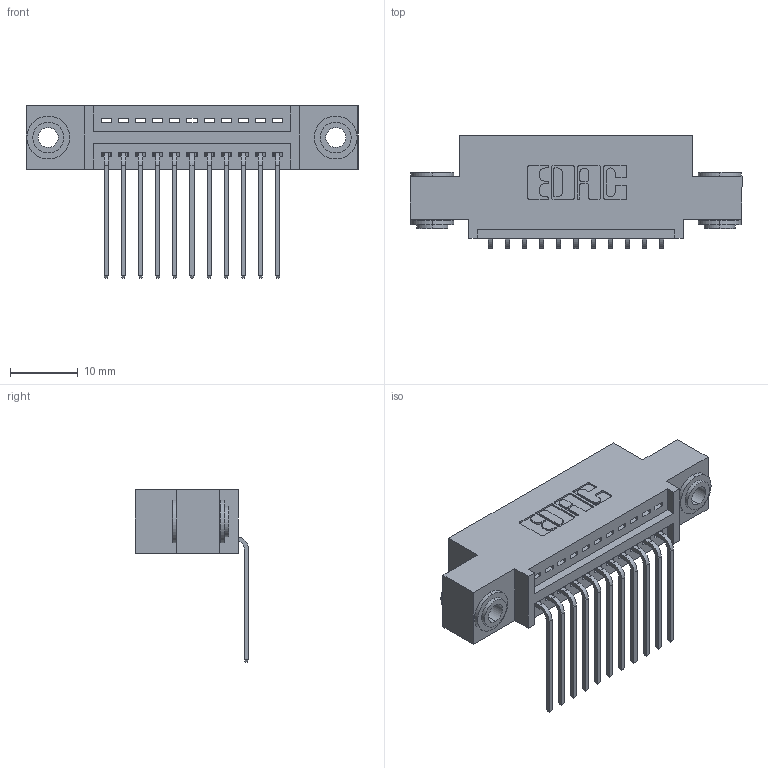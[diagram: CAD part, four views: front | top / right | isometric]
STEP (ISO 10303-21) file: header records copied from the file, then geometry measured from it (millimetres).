
FILE_DESCRIPTION (( 'STEP AP203' ), '1' );
FILE_NAME ('345-011-559-403.STEP', '2019-10-04T00:37:00', ( '' ), ( '' ), 'SwSTEP 2.0', 'SolidWorks 2016', '' );
FILE_SCHEMA (( 'CONFIG_CONTROL_DESIGN' ));
Length unit declared in the file: inch
Products named in the file (4): 345-292-001_558 559 Tail - 1; 345-011-559-403; 345-250-002_345-250-002-102; 345 Part_0.110 Offset - 0.156 Dia-TH
Assembly tree (14 placements, depth 2):
  345-011-559-403
    345 Part_0.110 Offset - 0.156 Dia-TH
    345-292-001_558 559 Tail - 1  x11
    345-250-002_345-250-002-102  x2
Bounding box: 49.15 x 16.75 x 25.53 mm (x, y, z)
Volume: 4397 mm3; surface area: 5933.6 mm2
Topology: 14 solids, 14 shells, 828 faces, 2431 edges, 1602 vertices
Faces by surface type: plane 556, cylinder 264, cone 8
Entity records: 13318 total; most frequent: CARTESIAN_POINT 2288, ORIENTED_EDGE 2226, DIRECTION 2073, EDGE_CURVE 1113, VECTOR 913, LINE 913, VERTEX_POINT 738, AXIS2_PLACEMENT_3D 580
